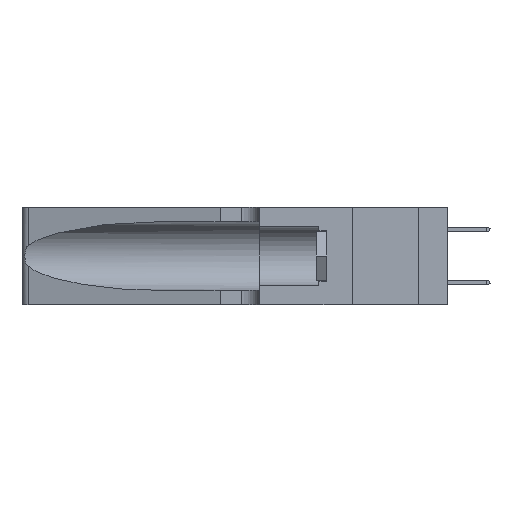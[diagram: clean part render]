
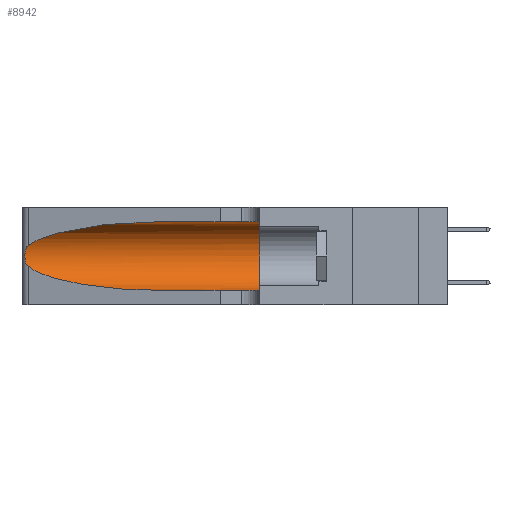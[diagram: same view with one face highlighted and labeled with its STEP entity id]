
A CAD part, left-side view. The second image highlights one B-rep face of the part: STEP entity #8942.
In plain terms, the highlighted cylindrical face has radius 3.308 mm (diameter 6.617 mm), a partial arc.
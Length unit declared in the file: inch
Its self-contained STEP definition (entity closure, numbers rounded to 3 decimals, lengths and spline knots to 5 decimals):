
#125 = CARTESIAN_POINT ( 'NONE',  ( 0.26075, 1.23896, 0.19203 ) ) ;
#1146 = ORIENTED_EDGE ( 'NONE', *, *, #21162, .T. ) ;
#1341 = CARTESIAN_POINT ( 'NONE',  ( 0.25487, 1.22718, 0.22369 ) ) ;
#1579 = CARTESIAN_POINT ( 'NONE',  ( 0.1305, 0.72297, 0.31525 ) ) ;
#1642 = CYLINDRICAL_SURFACE ( 'NONE', #18592, 0.13025 ) ;
#1660 = CARTESIAN_POINT ( 'NONE',  ( 0.25487, 1.22718, 0.22369 ) ) ;
#1887 = CARTESIAN_POINT ( 'NONE',  ( 0.25856, 1.23593, 0.16098 ) ) ;
#2496 = VECTOR ( 'NONE', #21102, 39.37008 ) ;
#2585 = DIRECTION ( 'NONE',  ( 0., 0., -1. ) ) ;
#2778 = VERTEX_POINT ( 'NONE', #19586 ) ;
#3838 = CARTESIAN_POINT ( 'NONE',  ( 0.1305, 0.72297, 0.31525 ) ) ;
#4030 = EDGE_CURVE ( 'NONE', #12924, #10402, #6887, .T. ) ;
#4552 = ORIENTED_EDGE ( 'NONE', *, *, #4030, .T. ) ;
#5106 = CARTESIAN_POINT ( 'NONE',  ( 0.25787, 1.23484, 0.2124 ) ) ;
#5406 = CARTESIAN_POINT ( 'NONE',  ( 0.25789, 1.23486, 0.15765 ) ) ;
#6487 = EDGE_CURVE ( 'NONE', #10402, #11174, #18561, .T. ) ;
#6521 = VERTEX_POINT ( 'NONE', #12473 ) ;
#6887 =( BOUNDED_CURVE ( )  B_SPLINE_CURVE ( 3, ( #1579, #8423, #13715, #1660 ),
 .UNSPECIFIED., .F., .F. ) 
 B_SPLINE_CURVE_WITH_KNOTS ( ( 4, 4 ),
 ( 1.5708, 2.84003 ),
 .UNSPECIFIED. ) 
 CURVE ( )  GEOMETRIC_REPRESENTATION_ITEM ( )  RATIONAL_B_SPLINE_CURVE ( ( 1., 0.87, 0.87, 1. ) ) 
 REPRESENTATION_ITEM ( '' )  );
#6925 = CARTESIAN_POINT ( 'NONE',  ( 0.26075, 1.23896, 0.178 ) ) ;
#7148 = CARTESIAN_POINT ( 'NONE',  ( 0.25487, 1.22718, 0.14631 ) ) ;
#8247 =( BOUNDED_CURVE ( )  B_SPLINE_CURVE ( 3, ( #14642, #15767, #17423, #8768 ),
 .UNSPECIFIED., .F., .F. ) 
 B_SPLINE_CURVE_WITH_KNOTS ( ( 4, 4 ),
 ( 3.44316, 4.71239 ),
 .UNSPECIFIED. ) 
 CURVE ( )  GEOMETRIC_REPRESENTATION_ITEM ( )  RATIONAL_B_SPLINE_CURVE ( ( 1., 0.87, 0.87, 1. ) ) 
 REPRESENTATION_ITEM ( '' )  );
#8325 = EDGE_CURVE ( 'NONE', #2778, #6521, #21871, .T. ) ;
#8368 = ORIENTED_EDGE ( 'NONE', *, *, #15647, .F. ) ;
#8423 = CARTESIAN_POINT ( 'NONE',  ( 0.18966, 0.96281, 0.31525 ) ) ;
#8667 = AXIS2_PLACEMENT_3D ( 'NONE', #9747, #19978, #19832 ) ;
#8768 = CARTESIAN_POINT ( 'NONE',  ( 0.1305, 0.72297, 0.05475 ) ) ;
#8798 = CARTESIAN_POINT ( 'NONE',  ( 0.25639, 1.23184, 0.21858 ) ) ;
#8942 = ADVANCED_FACE ( 'NONE', ( #14129 ), #1642, .F. ) ;
#9310 = VERTEX_POINT ( 'NONE', #17503 ) ;
#9747 = CARTESIAN_POINT ( 'NONE',  ( 0.1305, 0.35, 0.185 ) ) ;
#10369 = CARTESIAN_POINT ( 'NONE',  ( 0.26017, 1.23833, 0.17102 ) ) ;
#10402 = VERTEX_POINT ( 'NONE', #17359 ) ;
#10521 = CARTESIAN_POINT ( 'NONE',  ( 0.25854, 1.2359, 0.20912 ) ) ;
#10795 = CARTESIAN_POINT ( 'NONE',  ( 0.1305, 1.61858, 0.31525 ) ) ;
#10808 = DIRECTION ( 'NONE',  ( 0., -1., 0. ) ) ;
#11174 = VERTEX_POINT ( 'NONE', #12433 ) ;
#11939 = VECTOR ( 'NONE', #17581, 39.37008 ) ;
#12023 = CARTESIAN_POINT ( 'NONE',  ( 0.26018, 1.23835, 0.19895 ) ) ;
#12099 = CARTESIAN_POINT ( 'NONE',  ( 0.25639, 1.23186, 0.15144 ) ) ;
#12433 = CARTESIAN_POINT ( 'NONE',  ( 0.25487, 1.22718, 0.14631 ) ) ;
#12473 = CARTESIAN_POINT ( 'NONE',  ( 0.1305, 0.35, 0.05475 ) ) ;
#12924 = VERTEX_POINT ( 'NONE', #3838 ) ;
#13358 = LINE ( 'NONE', #14243, #2496 ) ;
#13475 = ORIENTED_EDGE ( 'NONE', *, *, #17687, .T. ) ;
#13715 = CARTESIAN_POINT ( 'NONE',  ( 0.2373, 1.15595, 0.28018 ) ) ;
#14129 = FACE_OUTER_BOUND ( 'NONE', #15761, .T. ) ;
#14243 = CARTESIAN_POINT ( 'NONE',  ( 0.1305, 1.61858, 0.05475 ) ) ;
#14642 = CARTESIAN_POINT ( 'NONE',  ( 0.25487, 1.22718, 0.14631 ) ) ;
#15647 = EDGE_CURVE ( 'NONE', #12924, #2778, #16509, .T. ) ;
#15761 = EDGE_LOOP ( 'NONE', ( #4552, #15829, #13475, #1146, #19656, #8368 ) ) ;
#15767 = CARTESIAN_POINT ( 'NONE',  ( 0.2373, 1.15595, 0.08982 ) ) ;
#15829 = ORIENTED_EDGE ( 'NONE', *, *, #6487, .T. ) ;
#16509 = LINE ( 'NONE', #10795, #11939 ) ;
#17218 = CARTESIAN_POINT ( 'NONE',  ( 0.25555, 1.22994, 0.2215 ) ) ;
#17293 = CARTESIAN_POINT ( 'NONE',  ( 0.25555, 1.22993, 0.14849 ) ) ;
#17359 = CARTESIAN_POINT ( 'NONE',  ( 0.25487, 1.22718, 0.22369 ) ) ;
#17423 = CARTESIAN_POINT ( 'NONE',  ( 0.18966, 0.96281, 0.05475 ) ) ;
#17503 = CARTESIAN_POINT ( 'NONE',  ( 0.1305, 0.72297, 0.05475 ) ) ;
#17581 = DIRECTION ( 'NONE',  ( 0., -1., 0. ) ) ;
#17599 = CARTESIAN_POINT ( 'NONE',  ( 0.1305, 1.61858, 0.185 ) ) ;
#17687 = EDGE_CURVE ( 'NONE', #11174, #9310, #8247, .T. ) ;
#18561 = B_SPLINE_CURVE_WITH_KNOTS ( 'NONE', 3,
 ( #1341, #17218, #8798, #5106, #10521, #12023, #125, #6925, #10369, #1887, #5406, #12099, #17293, #7148 ),
 .UNSPECIFIED., .F., .F.,
 ( 4, 2, 2, 2, 2, 2, 4 ),
 ( 0., 0.00027, 0.00053, 0.00107, 0.0016, 0.00187, 0.00214 ),
 .UNSPECIFIED. ) ;
#18592 = AXIS2_PLACEMENT_3D ( 'NONE', #17599, #10808, #2585 ) ;
#19586 = CARTESIAN_POINT ( 'NONE',  ( 0.1305, 0.35, 0.31525 ) ) ;
#19656 = ORIENTED_EDGE ( 'NONE', *, *, #8325, .F. ) ;
#19832 = DIRECTION ( 'NONE',  ( 0., 0., 1. ) ) ;
#19978 = DIRECTION ( 'NONE',  ( 0., 1., 0. ) ) ;
#21102 = DIRECTION ( 'NONE',  ( 0., -1., 0. ) ) ;
#21162 = EDGE_CURVE ( 'NONE', #9310, #6521, #13358, .T. ) ;
#21871 = CIRCLE ( 'NONE', #8667, 0.13025 ) ;
